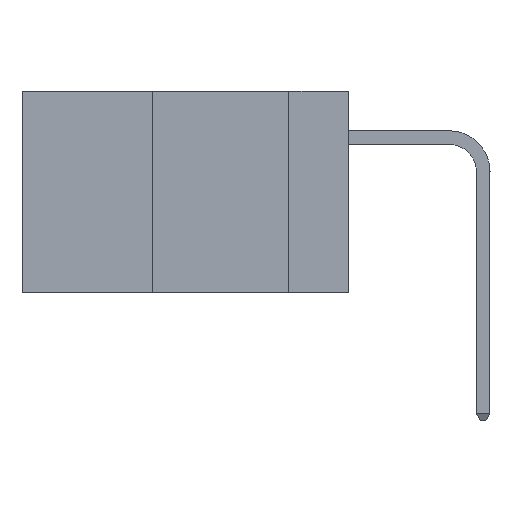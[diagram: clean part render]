
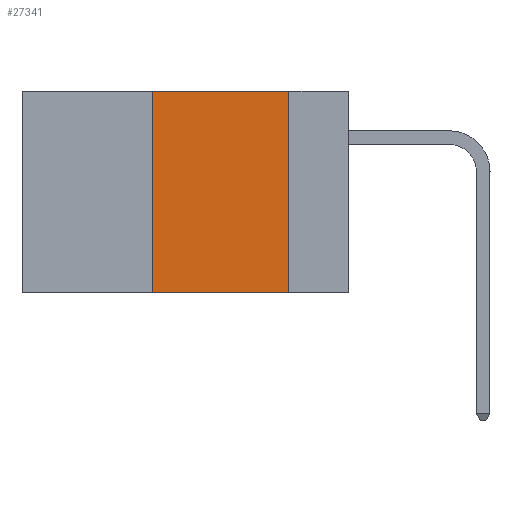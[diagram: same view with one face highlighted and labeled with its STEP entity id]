
A CAD part, left-side view. The second image highlights one B-rep face of the part: STEP entity #27341.
In plain terms, the highlighted planar face has unit normal (-1, 0, 0).
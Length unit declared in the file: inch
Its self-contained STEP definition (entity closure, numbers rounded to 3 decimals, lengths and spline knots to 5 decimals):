
#1117 = VERTEX_POINT ( 'NONE', #27906 ) ;
#1517 = VECTOR ( 'NONE', #4979, 39.37008 ) ;
#2382 = LINE ( 'NONE', #26281, #14536 ) ;
#4589 = CARTESIAN_POINT ( 'NONE',  ( 0., 0.11, 0. ) ) ;
#4979 = DIRECTION ( 'NONE',  ( 0., 0., -1. ) ) ;
#5176 = ORIENTED_EDGE ( 'NONE', *, *, #23781, .F. ) ;
#8226 = CARTESIAN_POINT ( 'NONE',  ( 0., 0.36, 0. ) ) ;
#9492 = ORIENTED_EDGE ( 'NONE', *, *, #28851, .F. ) ;
#14536 = VECTOR ( 'NONE', #20004, 39.37008 ) ;
#16135 = EDGE_CURVE ( 'NONE', #30491, #1117, #2382, .T. ) ;
#17202 = CARTESIAN_POINT ( 'NONE',  ( 0., 0.36, -0.37 ) ) ;
#19116 = EDGE_LOOP ( 'NONE', ( #29128, #9492, #5176, #28019 ) ) ;
#20004 = DIRECTION ( 'NONE',  ( 0., -1., 0. ) ) ;
#20423 = EDGE_CURVE ( 'NONE', #25430, #1117, #25307, .T. ) ;
#21386 = DIRECTION ( 'NONE',  ( 1., 0., 0. ) ) ;
#22360 = AXIS2_PLACEMENT_3D ( 'NONE', #36082, #21386, #32825 ) ;
#22663 = VECTOR ( 'NONE', #38289, 39.37008 ) ;
#23377 = VECTOR ( 'NONE', #29573, 39.37008 ) ;
#23781 = EDGE_CURVE ( 'NONE', #30491, #26149, #30577, .T. ) ;
#23814 = CARTESIAN_POINT ( 'NONE',  ( 0., 0.6, 0. ) ) ;
#25307 = LINE ( 'NONE', #4589, #1517 ) ;
#25430 = VERTEX_POINT ( 'NONE', #26167 ) ;
#26149 = VERTEX_POINT ( 'NONE', #8226 ) ;
#26167 = CARTESIAN_POINT ( 'NONE',  ( 0., 0.11, 0. ) ) ;
#26281 = CARTESIAN_POINT ( 'NONE',  ( 0., 0.6, -0.37 ) ) ;
#27341 = ADVANCED_FACE ( 'NONE', ( #28175 ), #33208, .F. ) ;
#27906 = CARTESIAN_POINT ( 'NONE',  ( 0., 0.11, -0.37 ) ) ;
#28019 = ORIENTED_EDGE ( 'NONE', *, *, #16135, .T. ) ;
#28175 = FACE_OUTER_BOUND ( 'NONE', #19116, .T. ) ;
#28851 = EDGE_CURVE ( 'NONE', #26149, #25430, #33125, .T. ) ;
#29128 = ORIENTED_EDGE ( 'NONE', *, *, #20423, .F. ) ;
#29573 = DIRECTION ( 'NONE',  ( 0., -1., 0. ) ) ;
#30491 = VERTEX_POINT ( 'NONE', #17202 ) ;
#30577 = LINE ( 'NONE', #35256, #22663 ) ;
#32825 = DIRECTION ( 'NONE',  ( 0., 0., -1. ) ) ;
#33125 = LINE ( 'NONE', #23814, #23377 ) ;
#33208 = PLANE ( 'NONE',  #22360 ) ;
#35256 = CARTESIAN_POINT ( 'NONE',  ( 0., 0.36, 0. ) ) ;
#36082 = CARTESIAN_POINT ( 'NONE',  ( 0., 0.6, 0. ) ) ;
#38289 = DIRECTION ( 'NONE',  ( 0., 0., 1. ) ) ;
